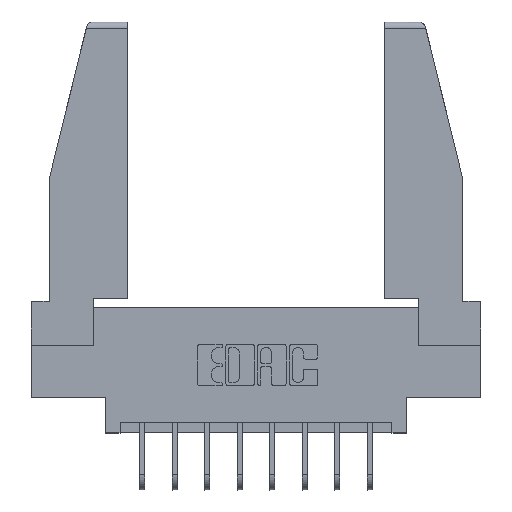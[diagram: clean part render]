
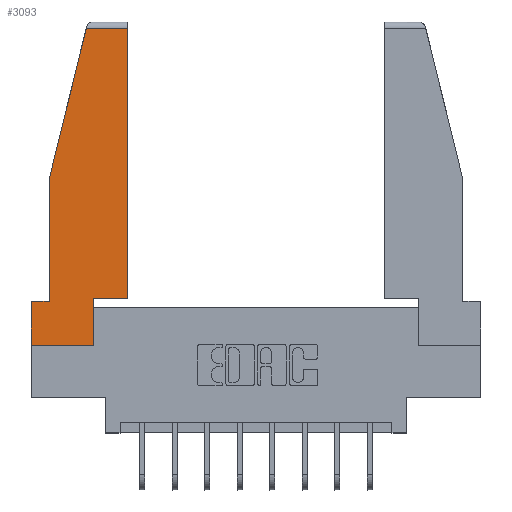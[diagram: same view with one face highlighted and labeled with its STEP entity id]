
A CAD part, top view. The second image highlights one B-rep face of the part: STEP entity #3093.
In plain terms, the highlighted planar face has unit normal (0, 0, 1).
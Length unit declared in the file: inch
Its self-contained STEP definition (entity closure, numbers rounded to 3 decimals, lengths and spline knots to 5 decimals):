
#85 = VECTOR ( 'NONE', #8896, 39.37008 ) ;
#114 = VERTEX_POINT ( 'NONE', #6666 ) ;
#864 = LINE ( 'NONE', #13781, #3612 ) ;
#982 = LINE ( 'NONE', #6530, #85 ) ;
#1347 = VECTOR ( 'NONE', #7088, 39.37008 ) ;
#1624 = ORIENTED_EDGE ( 'NONE', *, *, #13722, .T. ) ;
#1707 = CARTESIAN_POINT ( 'NONE',  ( 0., 1.52, 0. ) ) ;
#1828 = EDGE_CURVE ( 'NONE', #13732, #11456, #7172, .T. ) ;
#2206 = EDGE_CURVE ( 'NONE', #114, #6019, #8968, .T. ) ;
#2249 = CARTESIAN_POINT ( 'NONE',  ( 0.461, 0.223, 0. ) ) ;
#2355 = ORIENTED_EDGE ( 'NONE', *, *, #2735, .T. ) ;
#2593 = DIRECTION ( 'NONE',  ( 1., 0., 0. ) ) ;
#2602 = DIRECTION ( 'NONE',  ( 0., -1., 0. ) ) ;
#2665 = EDGE_CURVE ( 'NONE', #7262, #114, #8242, .T. ) ;
#2735 = EDGE_CURVE ( 'NONE', #6019, #13732, #8589, .T. ) ;
#2872 = ORIENTED_EDGE ( 'NONE', *, *, #14695, .T. ) ;
#2976 = VERTEX_POINT ( 'NONE', #14297 ) ;
#3093 = ADVANCED_FACE ( 'NONE', ( #13360 ), #12362, .T. ) ;
#3213 = LINE ( 'NONE', #8372, #8093 ) ;
#3612 = VECTOR ( 'NONE', #2593, 39.37008 ) ;
#3623 = CARTESIAN_POINT ( 'NONE',  ( 0., 0.21, 0. ) ) ;
#3768 = ORIENTED_EDGE ( 'NONE', *, *, #9303, .T. ) ;
#4244 = VECTOR ( 'NONE', #9832, 39.37008 ) ;
#5130 = CARTESIAN_POINT ( 'NONE',  ( 0.297, 0.223, 0. ) ) ;
#6019 = VERTEX_POINT ( 'NONE', #8681 ) ;
#6350 = ORIENTED_EDGE ( 'NONE', *, *, #1828, .T. ) ;
#6530 = CARTESIAN_POINT ( 'NONE',  ( 0.461, 0.223, 0. ) ) ;
#6577 = CARTESIAN_POINT ( 'NONE',  ( 0., 0.21, 0. ) ) ;
#6666 = CARTESIAN_POINT ( 'NONE',  ( 0.086, 0.8, 0. ) ) ;
#6734 = ORIENTED_EDGE ( 'NONE', *, *, #10279, .T. ) ;
#6832 = CARTESIAN_POINT ( 'NONE',  ( 0.297, 0.223, 0. ) ) ;
#6980 = ORIENTED_EDGE ( 'NONE', *, *, #2665, .T. ) ;
#7088 = DIRECTION ( 'NONE',  ( -0.239, -0.971, 0. ) ) ;
#7172 = LINE ( 'NONE', #10761, #8982 ) ;
#7262 = VERTEX_POINT ( 'NONE', #10785 ) ;
#7398 = CARTESIAN_POINT ( 'NONE',  ( 0., 0., 0. ) ) ;
#7924 = DIRECTION ( 'NONE',  ( 0., 0., 1. ) ) ;
#7984 = DIRECTION ( 'NONE',  ( 1., 0., 0. ) ) ;
#8093 = VECTOR ( 'NONE', #14223, 39.37008 ) ;
#8242 = LINE ( 'NONE', #9415, #1347 ) ;
#8372 = CARTESIAN_POINT ( 'NONE',  ( 0.297, 0., 0. ) ) ;
#8426 = ORIENTED_EDGE ( 'NONE', *, *, #12834, .T. ) ;
#8589 = LINE ( 'NONE', #3623, #10929 ) ;
#8600 = ORIENTED_EDGE ( 'NONE', *, *, #2206, .T. ) ;
#8681 = CARTESIAN_POINT ( 'NONE',  ( 0.086, 0.21, 0. ) ) ;
#8782 = CARTESIAN_POINT ( 'NONE',  ( 0.297, 0., 0. ) ) ;
#8896 = DIRECTION ( 'NONE',  ( 0., 1., 0. ) ) ;
#8968 = LINE ( 'NONE', #12864, #10402 ) ;
#8982 = VECTOR ( 'NONE', #10668, 39.37008 ) ;
#9303 = EDGE_CURVE ( 'NONE', #11456, #11974, #864, .T. ) ;
#9415 = CARTESIAN_POINT ( 'NONE',  ( 0.271, 1.55, 0. ) ) ;
#9832 = DIRECTION ( 'NONE',  ( -1., 0., 0. ) ) ;
#10279 = EDGE_CURVE ( 'NONE', #11974, #13847, #3213, .T. ) ;
#10402 = VECTOR ( 'NONE', #2602, 39.37008 ) ;
#10424 = DIRECTION ( 'NONE',  ( -1., 0., 0. ) ) ;
#10668 = DIRECTION ( 'NONE',  ( 0., -1., 0. ) ) ;
#10761 = CARTESIAN_POINT ( 'NONE',  ( 0., 0.21, 0. ) ) ;
#10785 = CARTESIAN_POINT ( 'NONE',  ( 0.2636, 1.52, 0. ) ) ;
#10929 = VECTOR ( 'NONE', #10424, 39.37008 ) ;
#11456 = VERTEX_POINT ( 'NONE', #7398 ) ;
#11891 = VERTEX_POINT ( 'NONE', #2249 ) ;
#11974 = VERTEX_POINT ( 'NONE', #8782 ) ;
#12043 = EDGE_LOOP ( 'NONE', ( #1624, #2872, #6980, #8600, #2355, #6350, #3768, #6734, #8426 ) ) ;
#12048 = LINE ( 'NONE', #5130, #13877 ) ;
#12362 = PLANE ( 'NONE',  #12591 ) ;
#12591 = AXIS2_PLACEMENT_3D ( 'NONE', #14897, #7924, #7984 ) ;
#12726 = LINE ( 'NONE', #1707, #4244 ) ;
#12834 = EDGE_CURVE ( 'NONE', #13847, #11891, #12048, .T. ) ;
#12864 = CARTESIAN_POINT ( 'NONE',  ( 0.086, 0.8, 0. ) ) ;
#13360 = FACE_OUTER_BOUND ( 'NONE', #12043, .T. ) ;
#13709 = DIRECTION ( 'NONE',  ( 1., 0., 0. ) ) ;
#13722 = EDGE_CURVE ( 'NONE', #11891, #2976, #982, .T. ) ;
#13732 = VERTEX_POINT ( 'NONE', #6577 ) ;
#13781 = CARTESIAN_POINT ( 'NONE',  ( 0., 0., 0. ) ) ;
#13847 = VERTEX_POINT ( 'NONE', #6832 ) ;
#13877 = VECTOR ( 'NONE', #13709, 39.37008 ) ;
#14223 = DIRECTION ( 'NONE',  ( 0., 1., 0. ) ) ;
#14297 = CARTESIAN_POINT ( 'NONE',  ( 0.461, 1.52, 0. ) ) ;
#14695 = EDGE_CURVE ( 'NONE', #2976, #7262, #12726, .T. ) ;
#14897 = CARTESIAN_POINT ( 'NONE',  ( 0., 0., 0. ) ) ;
